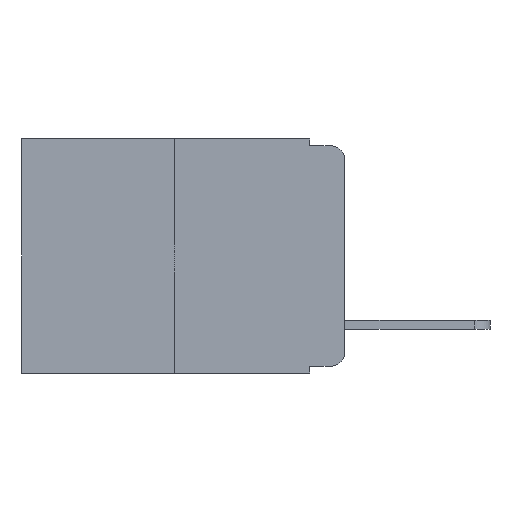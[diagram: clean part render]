
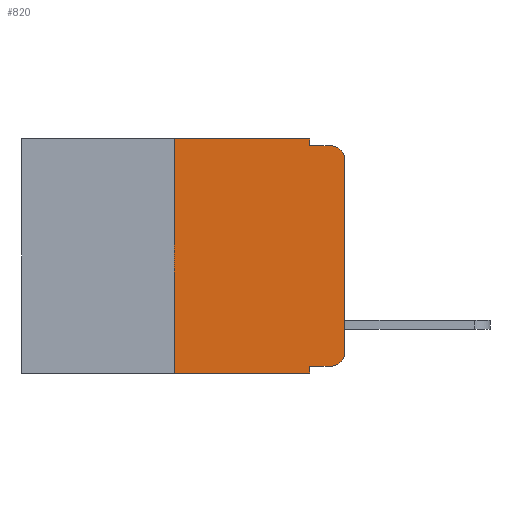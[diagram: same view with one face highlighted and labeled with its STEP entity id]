
A CAD part, left-side view. The second image highlights one B-rep face of the part: STEP entity #820.
In plain terms, the highlighted planar face has unit normal (-1, 0, 0).
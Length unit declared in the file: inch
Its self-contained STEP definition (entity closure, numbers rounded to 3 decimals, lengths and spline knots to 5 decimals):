
#34 = CARTESIAN_POINT ( 'NONE',  ( 0., 0.051, 0. ) ) ;
#280 = CARTESIAN_POINT ( 'NONE',  ( 0., 0.051, 0. ) ) ;
#321 = VERTEX_POINT ( 'NONE', #17490 ) ;
#323 = LINE ( 'NONE', #11467, #18960 ) ;
#538 = AXIS2_PLACEMENT_3D ( 'NONE', #17487, #9197, #18662 ) ;
#558 = FACE_OUTER_BOUND ( 'NONE', #15568, .T. ) ;
#582 = VERTEX_POINT ( 'NONE', #34 ) ;
#715 = CARTESIAN_POINT ( 'NONE',  ( 0., 0.051, -0.333 ) ) ;
#820 = ADVANCED_FACE ( 'NONE', ( #558 ), #1288, .F. ) ;
#840 = VERTEX_POINT ( 'NONE', #17226 ) ;
#1091 = CARTESIAN_POINT ( 'NONE',  ( 0., 0.473, 0. ) ) ;
#1288 = PLANE ( 'NONE',  #10577 ) ;
#1953 = VECTOR ( 'NONE', #10872, 39.37008 ) ;
#1956 = ORIENTED_EDGE ( 'NONE', *, *, #4614, .T. ) ;
#2301 = CARTESIAN_POINT ( 'NONE',  ( 0., 0.25, 0. ) ) ;
#2338 = VERTEX_POINT ( 'NONE', #3394 ) ;
#2397 = VECTOR ( 'NONE', #16084, 39.37008 ) ;
#2512 = ORIENTED_EDGE ( 'NONE', *, *, #4850, .T. ) ;
#2528 = DIRECTION ( 'NONE',  ( 0., 0., -1. ) ) ;
#2966 = DIRECTION ( 'NONE',  ( 0., 0., -1. ) ) ;
#3171 = VERTEX_POINT ( 'NONE', #14077 ) ;
#3394 = CARTESIAN_POINT ( 'NONE',  ( 0., 0.051, -0.01 ) ) ;
#3976 = VERTEX_POINT ( 'NONE', #15605 ) ;
#4137 = CARTESIAN_POINT ( 'NONE',  ( 0., 0., 0. ) ) ;
#4282 = VERTEX_POINT ( 'NONE', #11127 ) ;
#4369 = LINE ( 'NONE', #13145, #11749 ) ;
#4494 = EDGE_CURVE ( 'NONE', #321, #3171, #4369, .T. ) ;
#4614 = EDGE_CURVE ( 'NONE', #3976, #5929, #5613, .T. ) ;
#4650 = ORIENTED_EDGE ( 'NONE', *, *, #13998, .T. ) ;
#4850 = EDGE_CURVE ( 'NONE', #5929, #4282, #14998, .T. ) ;
#4855 = EDGE_CURVE ( 'NONE', #2338, #4282, #17697, .T. ) ;
#4959 = EDGE_CURVE ( 'NONE', #582, #2338, #8610, .T. ) ;
#5296 = EDGE_CURVE ( 'NONE', #321, #16176, #14331, .T. ) ;
#5613 = LINE ( 'NONE', #4137, #16555 ) ;
#5929 = VERTEX_POINT ( 'NONE', #6192 ) ;
#6192 = CARTESIAN_POINT ( 'NONE',  ( 0., 0., -0.03 ) ) ;
#6869 = ORIENTED_EDGE ( 'NONE', *, *, #4855, .F. ) ;
#7753 = ORIENTED_EDGE ( 'NONE', *, *, #5296, .F. ) ;
#8579 = DIRECTION ( 'NONE',  ( 0., 0., -1. ) ) ;
#8610 = LINE ( 'NONE', #280, #15696 ) ;
#9137 = ORIENTED_EDGE ( 'NONE', *, *, #13595, .T. ) ;
#9197 = DIRECTION ( 'NONE',  ( -1., 0., 0. ) ) ;
#9473 = CARTESIAN_POINT ( 'NONE',  ( 0., 0.051, 0. ) ) ;
#9534 = AXIS2_PLACEMENT_3D ( 'NONE', #14880, #12746, #8579 ) ;
#9817 = DIRECTION ( 'NONE',  ( 1., 0., 0. ) ) ;
#10577 = AXIS2_PLACEMENT_3D ( 'NONE', #1091, #9817, #2528 ) ;
#10872 = DIRECTION ( 'NONE',  ( 0., 0., -1. ) ) ;
#11127 = CARTESIAN_POINT ( 'NONE',  ( 0., 0.02, -0.01 ) ) ;
#11467 = CARTESIAN_POINT ( 'NONE',  ( 0., 0.051, -0.333 ) ) ;
#11749 = VECTOR ( 'NONE', #14909, 39.37008 ) ;
#11803 = EDGE_CURVE ( 'NONE', #16176, #582, #13572, .T. ) ;
#11840 = ORIENTED_EDGE ( 'NONE', *, *, #11803, .F. ) ;
#11876 = CARTESIAN_POINT ( 'NONE',  ( 0., 0.473, 0. ) ) ;
#12553 = DIRECTION ( 'NONE',  ( 0., -1., 0. ) ) ;
#12746 = DIRECTION ( 'NONE',  ( -1., 0., 0. ) ) ;
#12782 = CARTESIAN_POINT ( 'NONE',  ( 0., 0.051, -0.01 ) ) ;
#12877 = DIRECTION ( 'NONE',  ( 0., -1., 0. ) ) ;
#12973 = EDGE_CURVE ( 'NONE', #15439, #3171, #13967, .T. ) ;
#13145 = CARTESIAN_POINT ( 'NONE',  ( 0., 0.473, -0.343 ) ) ;
#13162 = DIRECTION ( 'NONE',  ( 0., 0., 1. ) ) ;
#13238 = CIRCLE ( 'NONE', #538, 0.02 ) ;
#13284 = DIRECTION ( 'NONE',  ( 0., -1., 0. ) ) ;
#13572 = LINE ( 'NONE', #11876, #16820 ) ;
#13595 = EDGE_CURVE ( 'NONE', #840, #3976, #13238, .T. ) ;
#13967 = LINE ( 'NONE', #9473, #1953 ) ;
#13998 = EDGE_CURVE ( 'NONE', #15439, #840, #323, .T. ) ;
#14077 = CARTESIAN_POINT ( 'NONE',  ( 0., 0.051, -0.343 ) ) ;
#14331 = LINE ( 'NONE', #2301, #2397 ) ;
#14414 = ORIENTED_EDGE ( 'NONE', *, *, #4959, .F. ) ;
#14578 = VECTOR ( 'NONE', #12553, 39.37008 ) ;
#14880 = CARTESIAN_POINT ( 'NONE',  ( 0., 0.02, -0.03 ) ) ;
#14909 = DIRECTION ( 'NONE',  ( 0., -1., 0. ) ) ;
#14998 = CIRCLE ( 'NONE', #9534, 0.02 ) ;
#15298 = ORIENTED_EDGE ( 'NONE', *, *, #4494, .T. ) ;
#15439 = VERTEX_POINT ( 'NONE', #715 ) ;
#15568 = EDGE_LOOP ( 'NONE', ( #1956, #2512, #6869, #14414, #11840, #7753, #15298, #18652, #4650, #9137 ) ) ;
#15605 = CARTESIAN_POINT ( 'NONE',  ( 0., 0., -0.313 ) ) ;
#15696 = VECTOR ( 'NONE', #2966, 39.37008 ) ;
#16084 = DIRECTION ( 'NONE',  ( 0., 0., 1. ) ) ;
#16176 = VERTEX_POINT ( 'NONE', #17672 ) ;
#16555 = VECTOR ( 'NONE', #13162, 39.37008 ) ;
#16820 = VECTOR ( 'NONE', #13284, 39.37008 ) ;
#17226 = CARTESIAN_POINT ( 'NONE',  ( 0., 0.02, -0.333 ) ) ;
#17487 = CARTESIAN_POINT ( 'NONE',  ( 0., 0.02, -0.313 ) ) ;
#17490 = CARTESIAN_POINT ( 'NONE',  ( 0., 0.25, -0.343 ) ) ;
#17672 = CARTESIAN_POINT ( 'NONE',  ( 0., 0.25, 0. ) ) ;
#17697 = LINE ( 'NONE', #12782, #14578 ) ;
#18652 = ORIENTED_EDGE ( 'NONE', *, *, #12973, .F. ) ;
#18662 = DIRECTION ( 'NONE',  ( 0., 0., -1. ) ) ;
#18960 = VECTOR ( 'NONE', #12877, 39.37008 ) ;
